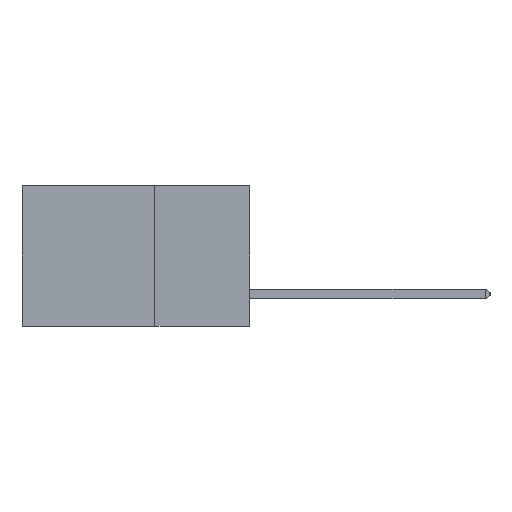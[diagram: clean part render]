
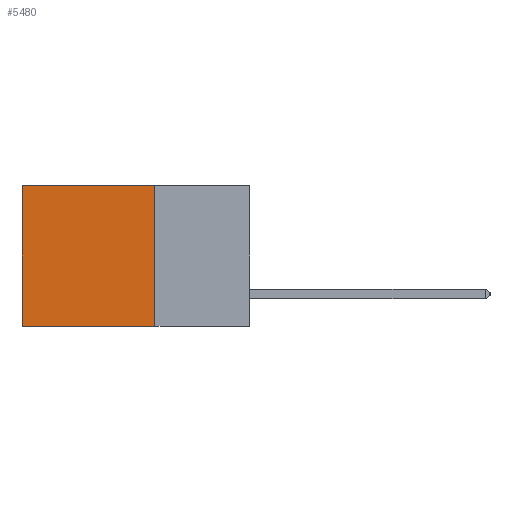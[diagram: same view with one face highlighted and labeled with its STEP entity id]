
A CAD part, left-side view. The second image highlights one B-rep face of the part: STEP entity #5480.
In plain terms, the highlighted planar face has unit normal (-1, 0, 0).
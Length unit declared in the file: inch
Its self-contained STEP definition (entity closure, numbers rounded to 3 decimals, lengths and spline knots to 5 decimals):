
#159 = VECTOR ( 'NONE', #9215, 39.37008 ) ;
#687 = CARTESIAN_POINT ( 'NONE',  ( 0.2875, 0.25, -0.37 ) ) ;
#756 = CARTESIAN_POINT ( 'NONE',  ( 0.2875, 0.25, -0.37 ) ) ;
#1084 = CARTESIAN_POINT ( 'NONE',  ( 0.2875, 0.6, -0.37 ) ) ;
#3316 = CARTESIAN_POINT ( 'NONE',  ( 0.2875, 0.25, 0. ) ) ;
#3525 = EDGE_LOOP ( 'NONE', ( #11319, #5799, #9127, #11409 ) ) ;
#3683 = DIRECTION ( 'NONE',  ( 0., 0., -1. ) ) ;
#3799 = VERTEX_POINT ( 'NONE', #13605 ) ;
#4359 = EDGE_CURVE ( 'NONE', #3799, #12168, #7185, .T. ) ;
#4469 = PLANE ( 'NONE',  #5322 ) ;
#5322 = AXIS2_PLACEMENT_3D ( 'NONE', #12856, #15563, #7361 ) ;
#5480 = ADVANCED_FACE ( 'NONE', ( #13966 ), #4469, .F. ) ;
#5799 = ORIENTED_EDGE ( 'NONE', *, *, #12140, .F. ) ;
#7185 = LINE ( 'NONE', #16093, #13648 ) ;
#7361 = DIRECTION ( 'NONE',  ( 0., 0., -1. ) ) ;
#9050 = VERTEX_POINT ( 'NONE', #1084 ) ;
#9127 = ORIENTED_EDGE ( 'NONE', *, *, #4359, .F. ) ;
#9215 = DIRECTION ( 'NONE',  ( 0., 1., 0. ) ) ;
#9299 = VERTEX_POINT ( 'NONE', #12770 ) ;
#9501 = VECTOR ( 'NONE', #10556, 39.37008 ) ;
#10144 = EDGE_CURVE ( 'NONE', #9299, #9050, #13165, .T. ) ;
#10556 = DIRECTION ( 'NONE',  ( 0., 0., -1. ) ) ;
#11319 = ORIENTED_EDGE ( 'NONE', *, *, #10144, .T. ) ;
#11409 = ORIENTED_EDGE ( 'NONE', *, *, #16659, .T. ) ;
#11908 = LINE ( 'NONE', #687, #159 ) ;
#12140 = EDGE_CURVE ( 'NONE', #12168, #9050, #11908, .T. ) ;
#12168 = VERTEX_POINT ( 'NONE', #756 ) ;
#12388 = LINE ( 'NONE', #3316, #12809 ) ;
#12770 = CARTESIAN_POINT ( 'NONE',  ( 0.2875, 0.6, 0. ) ) ;
#12809 = VECTOR ( 'NONE', #13079, 39.37008 ) ;
#12856 = CARTESIAN_POINT ( 'NONE',  ( 0.2875, 0.25, 0. ) ) ;
#13079 = DIRECTION ( 'NONE',  ( 0., 1., 0. ) ) ;
#13165 = LINE ( 'NONE', #14632, #9501 ) ;
#13605 = CARTESIAN_POINT ( 'NONE',  ( 0.2875, 0.25, 0. ) ) ;
#13648 = VECTOR ( 'NONE', #3683, 39.37008 ) ;
#13966 = FACE_OUTER_BOUND ( 'NONE', #3525, .T. ) ;
#14632 = CARTESIAN_POINT ( 'NONE',  ( 0.2875, 0.6, 0. ) ) ;
#15563 = DIRECTION ( 'NONE',  ( 1., 0., 0. ) ) ;
#16093 = CARTESIAN_POINT ( 'NONE',  ( 0.2875, 0.25, 0. ) ) ;
#16659 = EDGE_CURVE ( 'NONE', #3799, #9299, #12388, .T. ) ;
